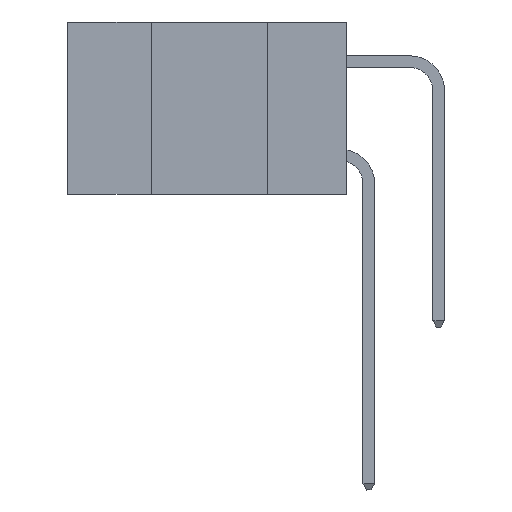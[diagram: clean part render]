
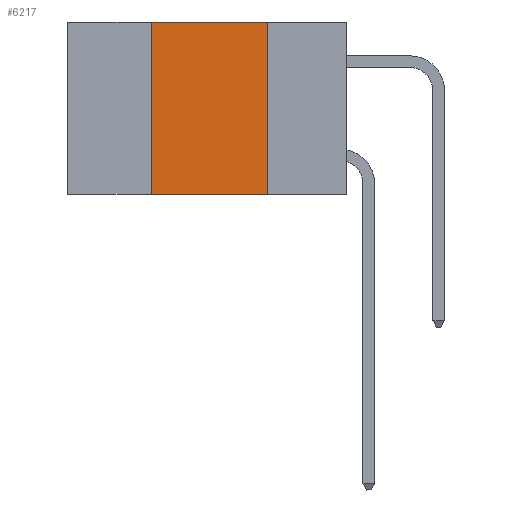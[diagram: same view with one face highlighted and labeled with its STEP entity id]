
A CAD part, left-side view. The second image highlights one B-rep face of the part: STEP entity #6217.
In plain terms, the highlighted planar face has unit normal (-1, 0, 0).
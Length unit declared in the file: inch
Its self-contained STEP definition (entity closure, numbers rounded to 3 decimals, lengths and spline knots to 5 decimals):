
#802 = DIRECTION ( 'NONE',  ( 0., 0., 1. ) ) ;
#1072 = DIRECTION ( 'NONE',  ( 0., 0., -1. ) ) ;
#1120 = VERTEX_POINT ( 'NONE', #8601 ) ;
#2038 = LINE ( 'NONE', #12919, #8735 ) ;
#2233 = CARTESIAN_POINT ( 'NONE',  ( 0., 0.6, -0.37 ) ) ;
#2237 = LINE ( 'NONE', #8655, #3107 ) ;
#2353 = DIRECTION ( 'NONE',  ( 0., -1., 0. ) ) ;
#2544 = ORIENTED_EDGE ( 'NONE', *, *, #15861, .T. ) ;
#2679 = VERTEX_POINT ( 'NONE', #7968 ) ;
#3082 = CARTESIAN_POINT ( 'NONE',  ( 0., 0.42, -0.37 ) ) ;
#3107 = VECTOR ( 'NONE', #12568, 39.37008 ) ;
#4978 = AXIS2_PLACEMENT_3D ( 'NONE', #12087, #7947, #1072 ) ;
#6217 = ADVANCED_FACE ( 'NONE', ( #8139 ), #9382, .F. ) ;
#6764 = CARTESIAN_POINT ( 'NONE',  ( 0., 0.17, 0. ) ) ;
#7947 = DIRECTION ( 'NONE',  ( 1., 0., 0. ) ) ;
#7968 = CARTESIAN_POINT ( 'NONE',  ( 0., 0.42, 0. ) ) ;
#8003 = LINE ( 'NONE', #2233, #9300 ) ;
#8139 = FACE_OUTER_BOUND ( 'NONE', #8155, .T. ) ;
#8155 = EDGE_LOOP ( 'NONE', ( #17025, #16581, #9540, #2544 ) ) ;
#8569 = VECTOR ( 'NONE', #802, 39.37008 ) ;
#8601 = CARTESIAN_POINT ( 'NONE',  ( 0., 0.17, -0.37 ) ) ;
#8655 = CARTESIAN_POINT ( 'NONE',  ( 0., 0.17, 0. ) ) ;
#8735 = VECTOR ( 'NONE', #10272, 39.37008 ) ;
#9300 = VECTOR ( 'NONE', #2353, 39.37008 ) ;
#9382 = PLANE ( 'NONE',  #4978 ) ;
#9540 = ORIENTED_EDGE ( 'NONE', *, *, #17654, .F. ) ;
#10272 = DIRECTION ( 'NONE',  ( 0., -1., 0. ) ) ;
#11711 = CARTESIAN_POINT ( 'NONE',  ( 0., 0.42, 0. ) ) ;
#12087 = CARTESIAN_POINT ( 'NONE',  ( 0., 0.6, 0. ) ) ;
#12568 = DIRECTION ( 'NONE',  ( 0., 0., -1. ) ) ;
#12919 = CARTESIAN_POINT ( 'NONE',  ( 0., 0.6, 0. ) ) ;
#13334 = EDGE_CURVE ( 'NONE', #2679, #17431, #2038, .T. ) ;
#13777 = EDGE_CURVE ( 'NONE', #17431, #1120, #2237, .T. ) ;
#15560 = VERTEX_POINT ( 'NONE', #3082 ) ;
#15861 = EDGE_CURVE ( 'NONE', #15560, #1120, #8003, .T. ) ;
#16259 = LINE ( 'NONE', #11711, #8569 ) ;
#16581 = ORIENTED_EDGE ( 'NONE', *, *, #13334, .F. ) ;
#17025 = ORIENTED_EDGE ( 'NONE', *, *, #13777, .F. ) ;
#17431 = VERTEX_POINT ( 'NONE', #6764 ) ;
#17654 = EDGE_CURVE ( 'NONE', #15560, #2679, #16259, .T. ) ;
